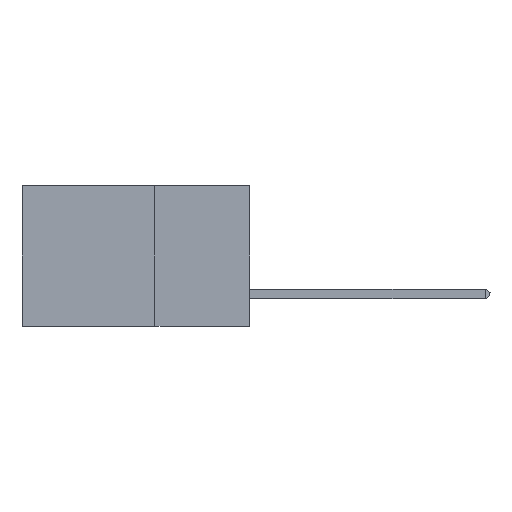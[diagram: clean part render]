
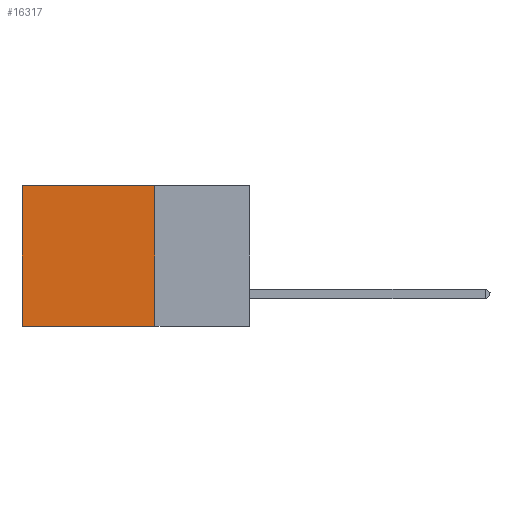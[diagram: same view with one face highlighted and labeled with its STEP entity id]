
A CAD part, left-side view. The second image highlights one B-rep face of the part: STEP entity #16317.
In plain terms, the highlighted planar face has unit normal (-1, 0, 0).
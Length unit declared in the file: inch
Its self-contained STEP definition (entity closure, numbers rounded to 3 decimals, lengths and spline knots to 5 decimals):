
#405 = EDGE_LOOP ( 'NONE', ( #20933, #6271, #11898, #3823 ) ) ;
#1758 = CARTESIAN_POINT ( 'NONE',  ( 0.2875, 0.25, 0. ) ) ;
#2871 = LINE ( 'NONE', #4348, #13973 ) ;
#3823 = ORIENTED_EDGE ( 'NONE', *, *, #8478, .T. ) ;
#4031 = EDGE_CURVE ( 'NONE', #17313, #7821, #9500, .T. ) ;
#4270 = DIRECTION ( 'NONE',  ( 0., 1., 0. ) ) ;
#4348 = CARTESIAN_POINT ( 'NONE',  ( 0.2875, 0.25, 0. ) ) ;
#4685 = EDGE_CURVE ( 'NONE', #18887, #7821, #10969, .T. ) ;
#5692 = VECTOR ( 'NONE', #9244, 39.37008 ) ;
#5992 = LINE ( 'NONE', #1758, #5692 ) ;
#6271 = ORIENTED_EDGE ( 'NONE', *, *, #4685, .F. ) ;
#7661 = AXIS2_PLACEMENT_3D ( 'NONE', #19663, #21307, #23198 ) ;
#7821 = VERTEX_POINT ( 'NONE', #12042 ) ;
#8134 = VERTEX_POINT ( 'NONE', #16119 ) ;
#8478 = EDGE_CURVE ( 'NONE', #8134, #17313, #2871, .T. ) ;
#8736 = CARTESIAN_POINT ( 'NONE',  ( 0.2875, 0.25, -0.37 ) ) ;
#8982 = FACE_OUTER_BOUND ( 'NONE', #405, .T. ) ;
#9199 = VECTOR ( 'NONE', #11187, 39.37008 ) ;
#9244 = DIRECTION ( 'NONE',  ( 0., 0., -1. ) ) ;
#9500 = LINE ( 'NONE', #10123, #16232 ) ;
#10123 = CARTESIAN_POINT ( 'NONE',  ( 0.2875, 0.6, 0. ) ) ;
#10969 = LINE ( 'NONE', #8736, #9199 ) ;
#11187 = DIRECTION ( 'NONE',  ( 0., 1., 0. ) ) ;
#11898 = ORIENTED_EDGE ( 'NONE', *, *, #17001, .F. ) ;
#12042 = CARTESIAN_POINT ( 'NONE',  ( 0.2875, 0.6, -0.37 ) ) ;
#13877 = DIRECTION ( 'NONE',  ( 0., 0., -1. ) ) ;
#13973 = VECTOR ( 'NONE', #4270, 39.37008 ) ;
#15889 = PLANE ( 'NONE',  #7661 ) ;
#16119 = CARTESIAN_POINT ( 'NONE',  ( 0.2875, 0.25, 0. ) ) ;
#16232 = VECTOR ( 'NONE', #13877, 39.37008 ) ;
#16317 = ADVANCED_FACE ( 'NONE', ( #8982 ), #15889, .F. ) ;
#17001 = EDGE_CURVE ( 'NONE', #8134, #18887, #5992, .T. ) ;
#17313 = VERTEX_POINT ( 'NONE', #20026 ) ;
#18887 = VERTEX_POINT ( 'NONE', #23397 ) ;
#19663 = CARTESIAN_POINT ( 'NONE',  ( 0.2875, 0.25, 0. ) ) ;
#20026 = CARTESIAN_POINT ( 'NONE',  ( 0.2875, 0.6, 0. ) ) ;
#20933 = ORIENTED_EDGE ( 'NONE', *, *, #4031, .T. ) ;
#21307 = DIRECTION ( 'NONE',  ( 1., 0., 0. ) ) ;
#23198 = DIRECTION ( 'NONE',  ( 0., 0., -1. ) ) ;
#23397 = CARTESIAN_POINT ( 'NONE',  ( 0.2875, 0.25, -0.37 ) ) ;
